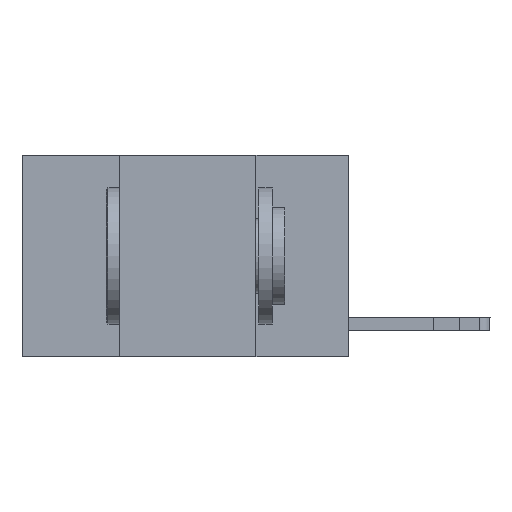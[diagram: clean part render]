
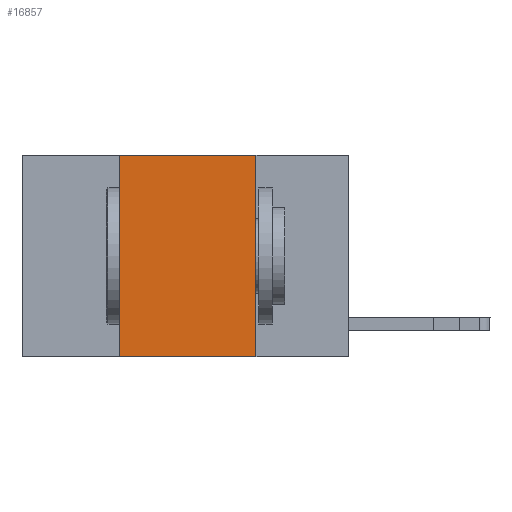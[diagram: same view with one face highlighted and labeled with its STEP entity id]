
A CAD part, left-side view. The second image highlights one B-rep face of the part: STEP entity #16857.
In plain terms, the highlighted planar face has unit normal (-1, 0, 0).
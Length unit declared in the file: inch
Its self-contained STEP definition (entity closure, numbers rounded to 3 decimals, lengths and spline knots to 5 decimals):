
#428 = CARTESIAN_POINT ( 'NONE',  ( 0., 0.6, 0. ) ) ;
#1746 = DIRECTION ( 'NONE',  ( 0., -1., 0. ) ) ;
#1875 = EDGE_CURVE ( 'NONE', #4332, #12111, #11601, .T. ) ;
#2301 = EDGE_CURVE ( 'NONE', #12111, #10019, #8414, .T. ) ;
#2660 = ORIENTED_EDGE ( 'NONE', *, *, #6103, .F. ) ;
#3101 = ORIENTED_EDGE ( 'NONE', *, *, #13816, .T. ) ;
#3519 = CARTESIAN_POINT ( 'NONE',  ( 0., 0.17, 0. ) ) ;
#3549 = CARTESIAN_POINT ( 'NONE',  ( 0., 0.6, 0. ) ) ;
#3651 = DIRECTION ( 'NONE',  ( 0., -1., 0. ) ) ;
#4332 = VERTEX_POINT ( 'NONE', #7034 ) ;
#5220 = FACE_OUTER_BOUND ( 'NONE', #7863, .T. ) ;
#5332 = DIRECTION ( 'NONE',  ( 1., 0., 0. ) ) ;
#6103 = EDGE_CURVE ( 'NONE', #15992, #4332, #12409, .T. ) ;
#6247 = CARTESIAN_POINT ( 'NONE',  ( 0., 0.17, 0. ) ) ;
#7034 = CARTESIAN_POINT ( 'NONE',  ( 0., 0.42, 0. ) ) ;
#7546 = VECTOR ( 'NONE', #11487, 39.37008 ) ;
#7821 = CARTESIAN_POINT ( 'NONE',  ( 0., 0.6, -0.37 ) ) ;
#7863 = EDGE_LOOP ( 'NONE', ( #8248, #18366, #2660, #3101 ) ) ;
#7987 = CARTESIAN_POINT ( 'NONE',  ( 0., 0.42, -0.37 ) ) ;
#8248 = ORIENTED_EDGE ( 'NONE', *, *, #2301, .F. ) ;
#8414 = LINE ( 'NONE', #3519, #7546 ) ;
#8495 = PLANE ( 'NONE',  #16680 ) ;
#10019 = VERTEX_POINT ( 'NONE', #17729 ) ;
#10824 = DIRECTION ( 'NONE',  ( 0., 0., 1. ) ) ;
#10935 = VECTOR ( 'NONE', #3651, 39.37008 ) ;
#11096 = VECTOR ( 'NONE', #10824, 39.37008 ) ;
#11487 = DIRECTION ( 'NONE',  ( 0., 0., -1. ) ) ;
#11601 = LINE ( 'NONE', #3549, #17848 ) ;
#12111 = VERTEX_POINT ( 'NONE', #6247 ) ;
#12409 = LINE ( 'NONE', #16875, #11096 ) ;
#13816 = EDGE_CURVE ( 'NONE', #15992, #10019, #15810, .T. ) ;
#15810 = LINE ( 'NONE', #7821, #10935 ) ;
#15992 = VERTEX_POINT ( 'NONE', #7987 ) ;
#16680 = AXIS2_PLACEMENT_3D ( 'NONE', #428, #5332, #16790 ) ;
#16790 = DIRECTION ( 'NONE',  ( 0., 0., -1. ) ) ;
#16857 = ADVANCED_FACE ( 'NONE', ( #5220 ), #8495, .F. ) ;
#16875 = CARTESIAN_POINT ( 'NONE',  ( 0., 0.42, 0. ) ) ;
#17729 = CARTESIAN_POINT ( 'NONE',  ( 0., 0.17, -0.37 ) ) ;
#17848 = VECTOR ( 'NONE', #1746, 39.37008 ) ;
#18366 = ORIENTED_EDGE ( 'NONE', *, *, #1875, .F. ) ;
